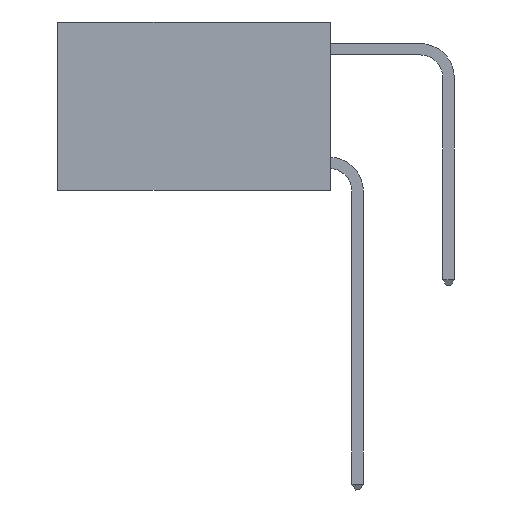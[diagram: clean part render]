
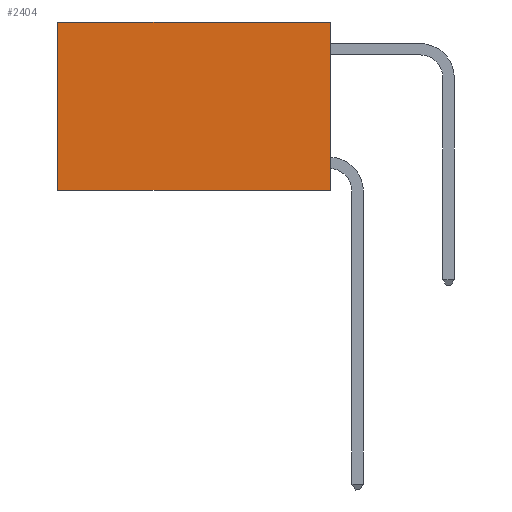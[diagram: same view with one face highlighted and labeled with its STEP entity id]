
A CAD part, left-side view. The second image highlights one B-rep face of the part: STEP entity #2404.
In plain terms, the highlighted planar face has unit normal (-1, 0, 0).
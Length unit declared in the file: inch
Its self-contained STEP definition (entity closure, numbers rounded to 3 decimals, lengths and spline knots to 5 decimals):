
#514 = CARTESIAN_POINT ( 'NONE',  ( 0.2625, 0., -0.37 ) ) ;
#531 = VECTOR ( 'NONE', #1449, 39.37008 ) ;
#596 = CARTESIAN_POINT ( 'NONE',  ( 0.2625, 0.6, 0. ) ) ;
#710 = DIRECTION ( 'NONE',  ( 0., 0., -1. ) ) ;
#752 = ORIENTED_EDGE ( 'NONE', *, *, #9264, .T. ) ;
#954 = VERTEX_POINT ( 'NONE', #4307 ) ;
#984 = VECTOR ( 'NONE', #5097, 39.37008 ) ;
#1277 = DIRECTION ( 'NONE',  ( 1., 0., 0. ) ) ;
#1449 = DIRECTION ( 'NONE',  ( 0., 1., 0. ) ) ;
#2404 = ADVANCED_FACE ( 'NONE', ( #5039 ), #2550, .F. ) ;
#2550 = PLANE ( 'NONE',  #5145 ) ;
#3280 = VECTOR ( 'NONE', #5425, 39.37008 ) ;
#3531 = CARTESIAN_POINT ( 'NONE',  ( 0.2625, 0., 0. ) ) ;
#3769 = LINE ( 'NONE', #10853, #984 ) ;
#4012 = CARTESIAN_POINT ( 'NONE',  ( 0.2625, 0., 0. ) ) ;
#4307 = CARTESIAN_POINT ( 'NONE',  ( 0.2625, 0.6, -0.37 ) ) ;
#4564 = CARTESIAN_POINT ( 'NONE',  ( 0.2625, 0.6, 0. ) ) ;
#4638 = VERTEX_POINT ( 'NONE', #7258 ) ;
#5039 = FACE_OUTER_BOUND ( 'NONE', #10632, .T. ) ;
#5097 = DIRECTION ( 'NONE',  ( 0., 1., 0. ) ) ;
#5145 = AXIS2_PLACEMENT_3D ( 'NONE', #4012, #1277, #710 ) ;
#5368 = LINE ( 'NONE', #6734, #531 ) ;
#5425 = DIRECTION ( 'NONE',  ( 0., 0., -1. ) ) ;
#5534 = LINE ( 'NONE', #4564, #3280 ) ;
#5902 = ORIENTED_EDGE ( 'NONE', *, *, #11050, .F. ) ;
#6734 = CARTESIAN_POINT ( 'NONE',  ( 0.2625, 0., 0. ) ) ;
#7107 = VERTEX_POINT ( 'NONE', #596 ) ;
#7258 = CARTESIAN_POINT ( 'NONE',  ( 0.2625, 0., 0. ) ) ;
#7724 = ORIENTED_EDGE ( 'NONE', *, *, #11173, .F. ) ;
#8498 = DIRECTION ( 'NONE',  ( 0., 0., -1. ) ) ;
#8816 = VECTOR ( 'NONE', #8498, 39.37008 ) ;
#9158 = ORIENTED_EDGE ( 'NONE', *, *, #10337, .T. ) ;
#9264 = EDGE_CURVE ( 'NONE', #7107, #954, #5534, .T. ) ;
#9354 = LINE ( 'NONE', #3531, #8816 ) ;
#10337 = EDGE_CURVE ( 'NONE', #4638, #7107, #5368, .T. ) ;
#10352 = VERTEX_POINT ( 'NONE', #514 ) ;
#10632 = EDGE_LOOP ( 'NONE', ( #752, #5902, #7724, #9158 ) ) ;
#10853 = CARTESIAN_POINT ( 'NONE',  ( 0.2625, 0., -0.37 ) ) ;
#11050 = EDGE_CURVE ( 'NONE', #10352, #954, #3769, .T. ) ;
#11173 = EDGE_CURVE ( 'NONE', #4638, #10352, #9354, .T. ) ;
